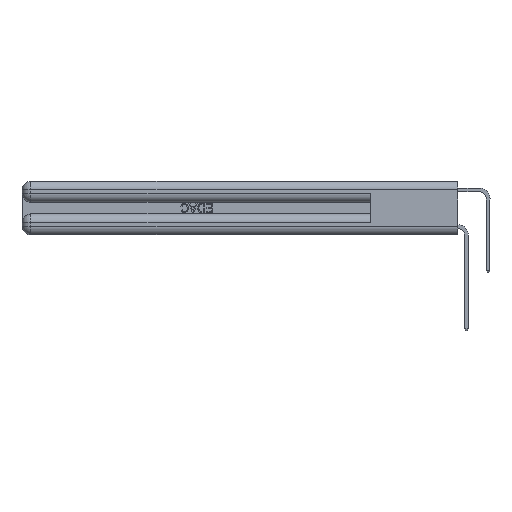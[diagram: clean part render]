
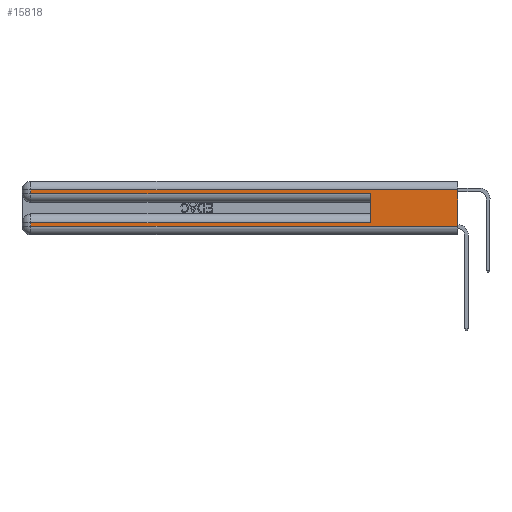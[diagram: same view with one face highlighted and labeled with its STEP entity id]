
A CAD part, left-side view. The second image highlights one B-rep face of the part: STEP entity #15818.
In plain terms, the highlighted planar face has unit normal (-1, 0, 0).
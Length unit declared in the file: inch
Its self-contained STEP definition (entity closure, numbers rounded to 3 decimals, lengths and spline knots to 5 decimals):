
#14 = EDGE_LOOP ( 'NONE', ( #7703, #17956, #277, #23948, #986, #17474, #1915, #27622 ) ) ;
#277 = ORIENTED_EDGE ( 'NONE', *, *, #19953, .T. ) ;
#668 = VECTOR ( 'NONE', #16207, 39.37008 ) ;
#861 = DIRECTION ( 'NONE',  ( 0., 1., 0. ) ) ;
#986 = ORIENTED_EDGE ( 'NONE', *, *, #10660, .F. ) ;
#1714 = VERTEX_POINT ( 'NONE', #14989 ) ;
#1915 = ORIENTED_EDGE ( 'NONE', *, *, #7541, .T. ) ;
#2004 = VERTEX_POINT ( 'NONE', #17990 ) ;
#2316 = VECTOR ( 'NONE', #24106, 39.37008 ) ;
#2442 = VECTOR ( 'NONE', #861, 39.37008 ) ;
#2475 = CARTESIAN_POINT ( 'NONE',  ( 0., 0., 0.31 ) ) ;
#3084 = LINE ( 'NONE', #8517, #8030 ) ;
#3662 = CARTESIAN_POINT ( 'NONE',  ( 0., 0., 0.37 ) ) ;
#4628 = EDGE_CURVE ( 'NONE', #17631, #2004, #23178, .T. ) ;
#6279 = LINE ( 'NONE', #24754, #25679 ) ;
#7427 = FACE_OUTER_BOUND ( 'NONE', #14, .T. ) ;
#7541 = EDGE_CURVE ( 'NONE', #22684, #1714, #10285, .T. ) ;
#7703 = ORIENTED_EDGE ( 'NONE', *, *, #11808, .F. ) ;
#8030 = VECTOR ( 'NONE', #21455, 39.37008 ) ;
#8517 = CARTESIAN_POINT ( 'NONE',  ( 0., 0., 0.06 ) ) ;
#8862 = DIRECTION ( 'NONE',  ( 0., 1., 0. ) ) ;
#8893 = VERTEX_POINT ( 'NONE', #15382 ) ;
#9323 = CARTESIAN_POINT ( 'NONE',  ( 0., 2.94, 0.285 ) ) ;
#9876 = AXIS2_PLACEMENT_3D ( 'NONE', #3662, #12433, #24871 ) ;
#10285 = LINE ( 'NONE', #12098, #668 ) ;
#10660 = EDGE_CURVE ( 'NONE', #24339, #8893, #20857, .T. ) ;
#11193 = CARTESIAN_POINT ( 'NONE',  ( 0., 0., 0.285 ) ) ;
#11404 = VECTOR ( 'NONE', #17796, 39.37008 ) ;
#11551 = EDGE_CURVE ( 'NONE', #27644, #8893, #24722, .T. ) ;
#11808 = EDGE_CURVE ( 'NONE', #17631, #12608, #6279, .T. ) ;
#11828 = VECTOR ( 'NONE', #8862, 39.37008 ) ;
#12098 = CARTESIAN_POINT ( 'NONE',  ( 0., 2.94, 0.37 ) ) ;
#12433 = DIRECTION ( 'NONE',  ( 1., 0., 0. ) ) ;
#12608 = VERTEX_POINT ( 'NONE', #14691 ) ;
#14319 = CARTESIAN_POINT ( 'NONE',  ( 0., 0., 0.31 ) ) ;
#14691 = CARTESIAN_POINT ( 'NONE',  ( 0., 0., 0.06 ) ) ;
#14989 = CARTESIAN_POINT ( 'NONE',  ( 0., 2.94, 0.06 ) ) ;
#15185 = DIRECTION ( 'NONE',  ( 0., 0., 1. ) ) ;
#15382 = CARTESIAN_POINT ( 'NONE',  ( 0., 0.6, 0.285 ) ) ;
#15818 = ADVANCED_FACE ( 'NONE', ( #7427 ), #20938, .F. ) ;
#16128 = EDGE_CURVE ( 'NONE', #24339, #22684, #23125, .T. ) ;
#16207 = DIRECTION ( 'NONE',  ( 0., 0., -1. ) ) ;
#16665 = EDGE_CURVE ( 'NONE', #1714, #12608, #3084, .T. ) ;
#17474 = ORIENTED_EDGE ( 'NONE', *, *, #16128, .T. ) ;
#17631 = VERTEX_POINT ( 'NONE', #14319 ) ;
#17796 = DIRECTION ( 'NONE',  ( 0., 0., -1. ) ) ;
#17956 = ORIENTED_EDGE ( 'NONE', *, *, #4628, .T. ) ;
#17990 = CARTESIAN_POINT ( 'NONE',  ( 0., 2.94, 0.31 ) ) ;
#19766 = CARTESIAN_POINT ( 'NONE',  ( 0., 2.94, 0.37 ) ) ;
#19953 = EDGE_CURVE ( 'NONE', #2004, #27644, #24449, .T. ) ;
#20206 = VECTOR ( 'NONE', #15185, 39.37008 ) ;
#20857 = LINE ( 'NONE', #21655, #20206 ) ;
#20938 = PLANE ( 'NONE',  #9876 ) ;
#21394 = CARTESIAN_POINT ( 'NONE',  ( 0., 2.94, 0.085 ) ) ;
#21455 = DIRECTION ( 'NONE',  ( 0., -1., 0. ) ) ;
#21655 = CARTESIAN_POINT ( 'NONE',  ( 0., 0.6, 0.145 ) ) ;
#22684 = VERTEX_POINT ( 'NONE', #21394 ) ;
#23125 = LINE ( 'NONE', #26628, #2442 ) ;
#23178 = LINE ( 'NONE', #2475, #11828 ) ;
#23948 = ORIENTED_EDGE ( 'NONE', *, *, #11551, .T. ) ;
#24106 = DIRECTION ( 'NONE',  ( 0., -1., 0. ) ) ;
#24159 = CARTESIAN_POINT ( 'NONE',  ( 0., 0.6, 0.085 ) ) ;
#24339 = VERTEX_POINT ( 'NONE', #24159 ) ;
#24449 = LINE ( 'NONE', #19766, #11404 ) ;
#24722 = LINE ( 'NONE', #11193, #2316 ) ;
#24754 = CARTESIAN_POINT ( 'NONE',  ( 0., 0., 0.37 ) ) ;
#24871 = DIRECTION ( 'NONE',  ( 0., 0., -1. ) ) ;
#25679 = VECTOR ( 'NONE', #26731, 39.37008 ) ;
#26628 = CARTESIAN_POINT ( 'NONE',  ( 0., 0., 0.085 ) ) ;
#26731 = DIRECTION ( 'NONE',  ( 0., 0., -1. ) ) ;
#27622 = ORIENTED_EDGE ( 'NONE', *, *, #16665, .T. ) ;
#27644 = VERTEX_POINT ( 'NONE', #9323 ) ;
